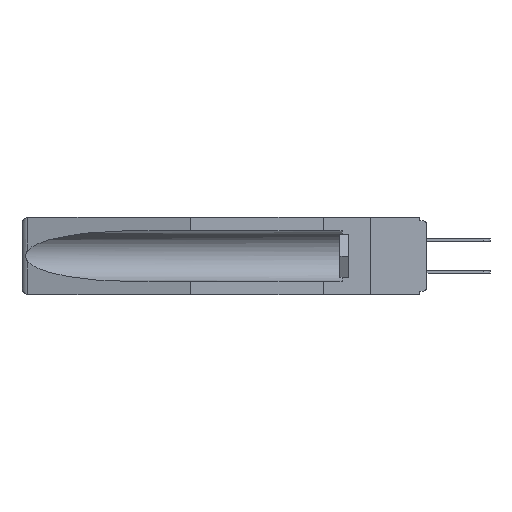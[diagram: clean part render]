
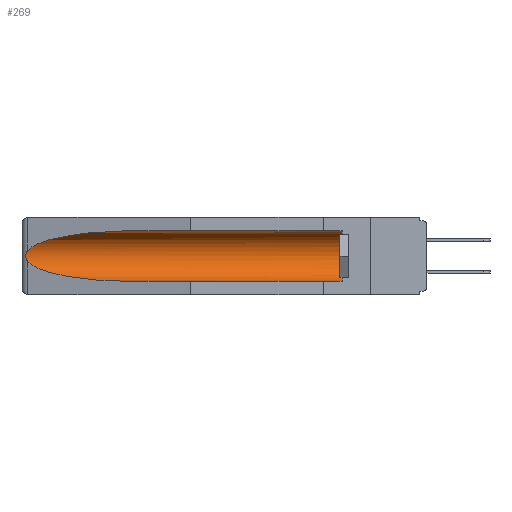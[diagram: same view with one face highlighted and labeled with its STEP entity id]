
A CAD part, left-side view. The second image highlights one B-rep face of the part: STEP entity #269.
In plain terms, the highlighted cylindrical face has radius 2.857 mm (diameter 5.715 mm), a partial arc.
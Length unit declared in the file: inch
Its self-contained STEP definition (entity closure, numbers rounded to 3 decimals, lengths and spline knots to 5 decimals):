
#46 =( BOUNDED_CURVE ( )  B_SPLINE_CURVE ( 3, ( #17531, #14001, #9229, #1088 ),
 .UNSPECIFIED., .F., .F. ) 
 B_SPLINE_CURVE_WITH_KNOTS ( ( 4, 4 ),
 ( 0.1948, 1.5708 ),
 .UNSPECIFIED. ) 
 CURVE ( )  GEOMETRIC_REPRESENTATION_ITEM ( )  RATIONAL_B_SPLINE_CURVE ( ( 1., 0.848, 0.848, 1. ) ) 
 REPRESENTATION_ITEM ( '' )  );
#216 = DIRECTION ( 'NONE',  ( 0., 0., 1. ) ) ;
#269 = ADVANCED_FACE ( 'NONE', ( #4923 ), #16622, .F. ) ;
#1088 = CARTESIAN_POINT ( 'NONE',  ( 0.155, 1.07973, -0.284 ) ) ;
#1717 = CARTESIAN_POINT ( 'NONE',  ( 0.2673, 1.5327, -0.16383 ) ) ;
#2128 = VERTEX_POINT ( 'NONE', #14218 ) ;
#3050 = VERTEX_POINT ( 'NONE', #19081 ) ;
#3319 = CARTESIAN_POINT ( 'NONE',  ( 0.26597, 1.5296, -0.19026 ) ) ;
#3393 = CARTESIAN_POINT ( 'NONE',  ( 0.26537, 1.52718, -0.19328 ) ) ;
#3564 = EDGE_CURVE ( 'NONE', #4450, #13336, #3819, .T. ) ;
#3819 = B_SPLINE_CURVE_WITH_KNOTS ( 'NONE', 3,
 ( #13142, #11359, #19658, #1717, #16245, #8078, #17822, #6518, #3319, #3393 ),
 .UNSPECIFIED., .F., .F.,
 ( 4, 2, 2, 2, 4 ),
 ( 0., 0.00029, 0.00058, 0.00087, 0.00117 ),
 .UNSPECIFIED. ) ;
#3912 = DIRECTION ( 'NONE',  ( 0., 0., 1. ) ) ;
#4101 = VERTEX_POINT ( 'NONE', #12545 ) ;
#4450 = VERTEX_POINT ( 'NONE', #12774 ) ;
#4923 = FACE_OUTER_BOUND ( 'NONE', #19372, .T. ) ;
#5518 = ORIENTED_EDGE ( 'NONE', *, *, #3564, .T. ) ;
#5757 = ORIENTED_EDGE ( 'NONE', *, *, #10632, .T. ) ;
#6518 = CARTESIAN_POINT ( 'NONE',  ( 0.26655, 1.53094, -0.18657 ) ) ;
#7066 =( BOUNDED_CURVE ( )  B_SPLINE_CURVE ( 3, ( #17517, #7771, #20782, #20497 ),
 .UNSPECIFIED., .F., .F. ) 
 B_SPLINE_CURVE_WITH_KNOTS ( ( 4, 4 ),
 ( 4.71239, 6.08839 ),
 .UNSPECIFIED. ) 
 CURVE ( )  GEOMETRIC_REPRESENTATION_ITEM ( )  RATIONAL_B_SPLINE_CURVE ( ( 1., 0.848, 0.848, 1. ) ) 
 REPRESENTATION_ITEM ( '' )  );
#7177 = CARTESIAN_POINT ( 'NONE',  ( 0.155, -0.30754, -0.1715 ) ) ;
#7190 = EDGE_CURVE ( 'NONE', #4101, #2128, #7477, .T. ) ;
#7340 = CIRCLE ( 'NONE', #16163, 0.1125 ) ;
#7477 = LINE ( 'NONE', #8057, #9268 ) ;
#7771 = CARTESIAN_POINT ( 'NONE',  ( 0.21114, 1.30732, -0.059 ) ) ;
#7972 = VECTOR ( 'NONE', #11306, 39.37008 ) ;
#7973 = CARTESIAN_POINT ( 'NONE',  ( 0.155, 0.126, -0.059 ) ) ;
#8057 = CARTESIAN_POINT ( 'NONE',  ( 0.155, -0.30754, -0.284 ) ) ;
#8078 = CARTESIAN_POINT ( 'NONE',  ( 0.2675, 1.53308, -0.17534 ) ) ;
#8749 = ORIENTED_EDGE ( 'NONE', *, *, #13862, .T. ) ;
#9229 = CARTESIAN_POINT ( 'NONE',  ( 0.21114, 1.30732, -0.284 ) ) ;
#9268 = VECTOR ( 'NONE', #16649, 39.37008 ) ;
#9870 = DIRECTION ( 'NONE',  ( 0., -1., 0. ) ) ;
#10249 = DIRECTION ( 'NONE',  ( 0., 1., 0. ) ) ;
#10430 = VERTEX_POINT ( 'NONE', #7973 ) ;
#10632 = EDGE_CURVE ( 'NONE', #4101, #10430, #7340, .T. ) ;
#10981 = EDGE_CURVE ( 'NONE', #13336, #2128, #46, .T. ) ;
#11168 = CARTESIAN_POINT ( 'NONE',  ( 0.155, -0.30754, -0.059 ) ) ;
#11276 = ORIENTED_EDGE ( 'NONE', *, *, #7190, .F. ) ;
#11306 = DIRECTION ( 'NONE',  ( 0., 1., 0. ) ) ;
#11359 = CARTESIAN_POINT ( 'NONE',  ( 0.26597, 1.52961, -0.15275 ) ) ;
#12072 = LINE ( 'NONE', #11168, #7972 ) ;
#12545 = CARTESIAN_POINT ( 'NONE',  ( 0.155, 0.126, -0.284 ) ) ;
#12774 = CARTESIAN_POINT ( 'NONE',  ( 0.26537, 1.52718, -0.14972 ) ) ;
#13142 = CARTESIAN_POINT ( 'NONE',  ( 0.26537, 1.52718, -0.14972 ) ) ;
#13336 = VERTEX_POINT ( 'NONE', #20670 ) ;
#13862 = EDGE_CURVE ( 'NONE', #3050, #4450, #7066, .T. ) ;
#14001 = CARTESIAN_POINT ( 'NONE',  ( 0.25451, 1.48313, -0.24835 ) ) ;
#14045 = ORIENTED_EDGE ( 'NONE', *, *, #20320, .T. ) ;
#14218 = CARTESIAN_POINT ( 'NONE',  ( 0.155, 1.07973, -0.284 ) ) ;
#15841 = ORIENTED_EDGE ( 'NONE', *, *, #10981, .T. ) ;
#16163 = AXIS2_PLACEMENT_3D ( 'NONE', #16252, #9870, #216 ) ;
#16245 = CARTESIAN_POINT ( 'NONE',  ( 0.2675, 1.53308, -0.16763 ) ) ;
#16252 = CARTESIAN_POINT ( 'NONE',  ( 0.155, 0.126, -0.1715 ) ) ;
#16622 = CYLINDRICAL_SURFACE ( 'NONE', #20068, 0.1125 ) ;
#16649 = DIRECTION ( 'NONE',  ( 0., 1., 0. ) ) ;
#17517 = CARTESIAN_POINT ( 'NONE',  ( 0.155, 1.07973, -0.059 ) ) ;
#17531 = CARTESIAN_POINT ( 'NONE',  ( 0.26537, 1.52718, -0.19328 ) ) ;
#17822 = CARTESIAN_POINT ( 'NONE',  ( 0.2673, 1.53269, -0.17917 ) ) ;
#19081 = CARTESIAN_POINT ( 'NONE',  ( 0.155, 1.07973, -0.059 ) ) ;
#19372 = EDGE_LOOP ( 'NONE', ( #8749, #5518, #15841, #11276, #5757, #14045 ) ) ;
#19658 = CARTESIAN_POINT ( 'NONE',  ( 0.26654, 1.53092, -0.15636 ) ) ;
#20068 = AXIS2_PLACEMENT_3D ( 'NONE', #7177, #10249, #3912 ) ;
#20320 = EDGE_CURVE ( 'NONE', #10430, #3050, #12072, .T. ) ;
#20497 = CARTESIAN_POINT ( 'NONE',  ( 0.26537, 1.52718, -0.14972 ) ) ;
#20670 = CARTESIAN_POINT ( 'NONE',  ( 0.26537, 1.52718, -0.19328 ) ) ;
#20782 = CARTESIAN_POINT ( 'NONE',  ( 0.25451, 1.48313, -0.09465 ) ) ;
